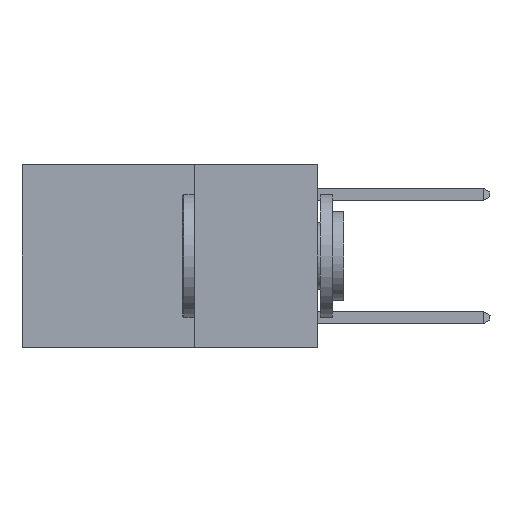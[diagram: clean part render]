
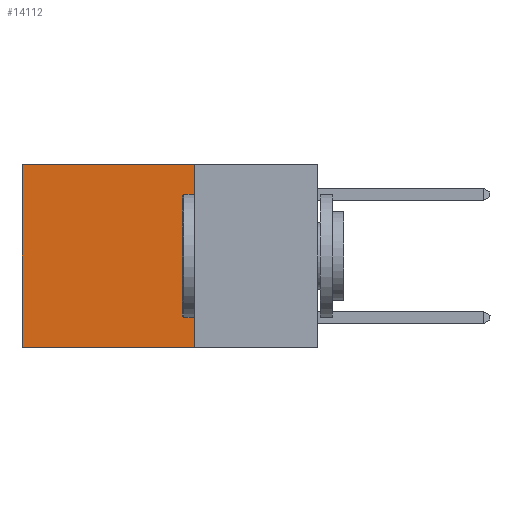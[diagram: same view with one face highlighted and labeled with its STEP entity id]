
A CAD part, left-side view. The second image highlights one B-rep face of the part: STEP entity #14112.
In plain terms, the highlighted planar face has unit normal (-1, 0, 0).
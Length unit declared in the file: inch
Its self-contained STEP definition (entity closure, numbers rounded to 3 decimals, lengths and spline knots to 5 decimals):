
#220 = VECTOR ( 'NONE', #11434, 39.37008 ) ;
#659 = ORIENTED_EDGE ( 'NONE', *, *, #11416, .F. ) ;
#1720 = ORIENTED_EDGE ( 'NONE', *, *, #13859, .F. ) ;
#2105 = VERTEX_POINT ( 'NONE', #4362 ) ;
#2666 = LINE ( 'NONE', #12069, #9701 ) ;
#3283 = DIRECTION ( 'NONE',  ( 0., 1., 0. ) ) ;
#3490 = AXIS2_PLACEMENT_3D ( 'NONE', #11216, #5545, #12452 ) ;
#3621 = CARTESIAN_POINT ( 'NONE',  ( 0.2625, 0.25, -0.37 ) ) ;
#3876 = LINE ( 'NONE', #4336, #11382 ) ;
#4336 = CARTESIAN_POINT ( 'NONE',  ( 0.2625, 0.25, 0. ) ) ;
#4362 = CARTESIAN_POINT ( 'NONE',  ( 0.2625, 0.6, 0. ) ) ;
#5545 = DIRECTION ( 'NONE',  ( 1., 0., 0. ) ) ;
#5663 = FACE_OUTER_BOUND ( 'NONE', #11287, .T. ) ;
#6073 = CARTESIAN_POINT ( 'NONE',  ( 0.2625, 0.25, 0. ) ) ;
#6292 = VERTEX_POINT ( 'NONE', #11985 ) ;
#6441 = ORIENTED_EDGE ( 'NONE', *, *, #10916, .T. ) ;
#6899 = PLANE ( 'NONE',  #3490 ) ;
#8653 = LINE ( 'NONE', #6073, #10518 ) ;
#9440 = DIRECTION ( 'NONE',  ( 0., 0., -1. ) ) ;
#9701 = VECTOR ( 'NONE', #11218, 39.37008 ) ;
#9774 = VERTEX_POINT ( 'NONE', #11288 ) ;
#10118 = LINE ( 'NONE', #3621, #220 ) ;
#10518 = VECTOR ( 'NONE', #9440, 39.37008 ) ;
#10916 = EDGE_CURVE ( 'NONE', #9774, #2105, #3876, .T. ) ;
#11216 = CARTESIAN_POINT ( 'NONE',  ( 0.2625, 0.25, 0. ) ) ;
#11218 = DIRECTION ( 'NONE',  ( 0., 0., -1. ) ) ;
#11287 = EDGE_LOOP ( 'NONE', ( #12608, #1720, #659, #6441 ) ) ;
#11288 = CARTESIAN_POINT ( 'NONE',  ( 0.2625, 0.25, 0. ) ) ;
#11382 = VECTOR ( 'NONE', #3283, 39.37008 ) ;
#11416 = EDGE_CURVE ( 'NONE', #9774, #11982, #8653, .T. ) ;
#11434 = DIRECTION ( 'NONE',  ( 0., 1., 0. ) ) ;
#11982 = VERTEX_POINT ( 'NONE', #13416 ) ;
#11985 = CARTESIAN_POINT ( 'NONE',  ( 0.2625, 0.6, -0.37 ) ) ;
#12069 = CARTESIAN_POINT ( 'NONE',  ( 0.2625, 0.6, 0. ) ) ;
#12452 = DIRECTION ( 'NONE',  ( 0., 0., -1. ) ) ;
#12608 = ORIENTED_EDGE ( 'NONE', *, *, #13153, .T. ) ;
#13153 = EDGE_CURVE ( 'NONE', #2105, #6292, #2666, .T. ) ;
#13416 = CARTESIAN_POINT ( 'NONE',  ( 0.2625, 0.25, -0.37 ) ) ;
#13859 = EDGE_CURVE ( 'NONE', #11982, #6292, #10118, .T. ) ;
#14112 = ADVANCED_FACE ( 'NONE', ( #5663 ), #6899, .F. ) ;
